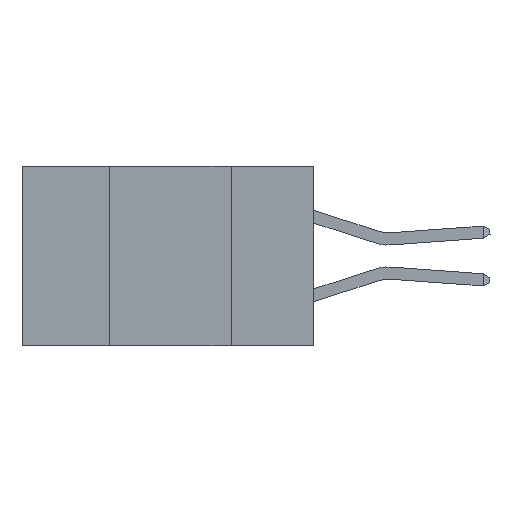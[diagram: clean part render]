
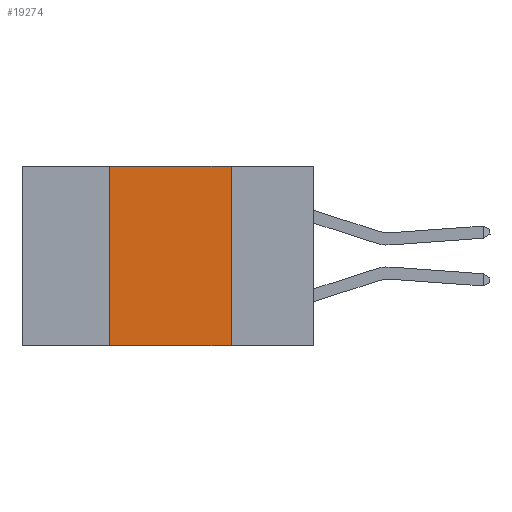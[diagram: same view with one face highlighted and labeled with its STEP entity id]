
A CAD part, left-side view. The second image highlights one B-rep face of the part: STEP entity #19274.
In plain terms, the highlighted planar face has unit normal (-1, 0, 0).
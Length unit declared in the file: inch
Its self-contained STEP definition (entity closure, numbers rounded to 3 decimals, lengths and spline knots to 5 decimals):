
#1962 = LINE ( 'NONE', #2404, #5227 ) ;
#2404 = CARTESIAN_POINT ( 'NONE',  ( 0., 0.6, 0. ) ) ;
#3049 = LINE ( 'NONE', #5205, #12521 ) ;
#3474 = VERTEX_POINT ( 'NONE', #12691 ) ;
#3758 = DIRECTION ( 'NONE',  ( 0., -1., 0. ) ) ;
#3902 = EDGE_CURVE ( 'NONE', #3474, #22543, #1962, .T. ) ;
#3948 = CARTESIAN_POINT ( 'NONE',  ( 0., 0.6, 0. ) ) ;
#4269 = VERTEX_POINT ( 'NONE', #7866 ) ;
#5205 = CARTESIAN_POINT ( 'NONE',  ( 0., 0.42, 0. ) ) ;
#5227 = VECTOR ( 'NONE', #18822, 39.37008 ) ;
#6720 = EDGE_LOOP ( 'NONE', ( #23193, #9675, #9674, #21225 ) ) ;
#7643 = VERTEX_POINT ( 'NONE', #20709 ) ;
#7866 = CARTESIAN_POINT ( 'NONE',  ( 0., 0.17, -0.37 ) ) ;
#8363 = PLANE ( 'NONE',  #14016 ) ;
#9674 = ORIENTED_EDGE ( 'NONE', *, *, #10893, .F. ) ;
#9675 = ORIENTED_EDGE ( 'NONE', *, *, #3902, .F. ) ;
#10457 = VECTOR ( 'NONE', #3758, 39.37008 ) ;
#10468 = DIRECTION ( 'NONE',  ( 0., 0., -1. ) ) ;
#10893 = EDGE_CURVE ( 'NONE', #7643, #3474, #3049, .T. ) ;
#12224 = VECTOR ( 'NONE', #14486, 39.37008 ) ;
#12521 = VECTOR ( 'NONE', #20080, 39.37008 ) ;
#12691 = CARTESIAN_POINT ( 'NONE',  ( 0., 0.42, 0. ) ) ;
#14016 = AXIS2_PLACEMENT_3D ( 'NONE', #3948, #23173, #10468 ) ;
#14130 = CARTESIAN_POINT ( 'NONE',  ( 0., 0.6, -0.37 ) ) ;
#14486 = DIRECTION ( 'NONE',  ( 0., 0., -1. ) ) ;
#18035 = CARTESIAN_POINT ( 'NONE',  ( 0., 0.17, 0. ) ) ;
#18606 = CARTESIAN_POINT ( 'NONE',  ( 0., 0.17, 0. ) ) ;
#18822 = DIRECTION ( 'NONE',  ( 0., -1., 0. ) ) ;
#19060 = EDGE_CURVE ( 'NONE', #7643, #4269, #24600, .T. ) ;
#19274 = ADVANCED_FACE ( 'NONE', ( #23948 ), #8363, .F. ) ;
#19476 = LINE ( 'NONE', #18606, #12224 ) ;
#20080 = DIRECTION ( 'NONE',  ( 0., 0., 1. ) ) ;
#20709 = CARTESIAN_POINT ( 'NONE',  ( 0., 0.42, -0.37 ) ) ;
#21225 = ORIENTED_EDGE ( 'NONE', *, *, #19060, .T. ) ;
#22543 = VERTEX_POINT ( 'NONE', #18035 ) ;
#22730 = EDGE_CURVE ( 'NONE', #22543, #4269, #19476, .T. ) ;
#23173 = DIRECTION ( 'NONE',  ( 1., 0., 0. ) ) ;
#23193 = ORIENTED_EDGE ( 'NONE', *, *, #22730, .F. ) ;
#23948 = FACE_OUTER_BOUND ( 'NONE', #6720, .T. ) ;
#24600 = LINE ( 'NONE', #14130, #10457 ) ;
